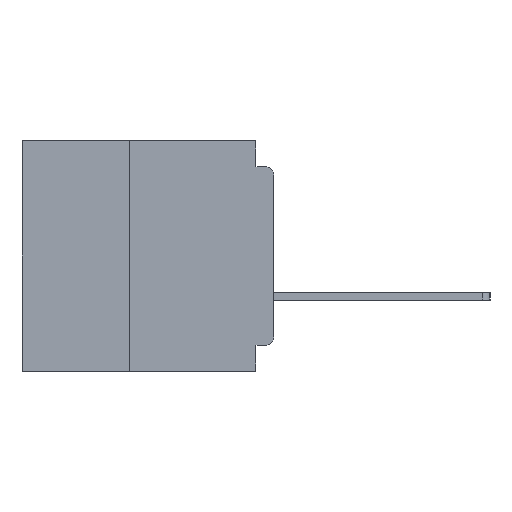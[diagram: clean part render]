
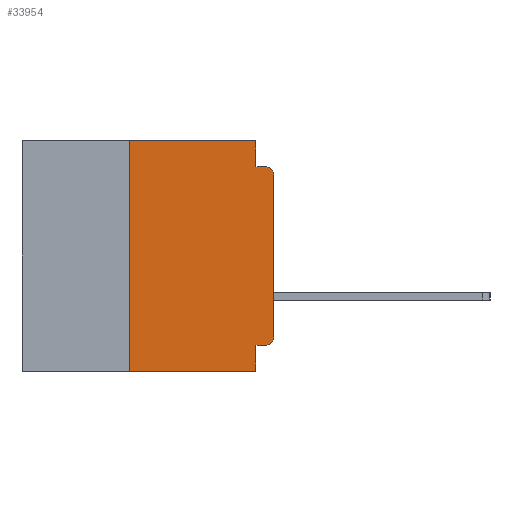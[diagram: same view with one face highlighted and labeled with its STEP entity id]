
A CAD part, left-side view. The second image highlights one B-rep face of the part: STEP entity #33954.
In plain terms, the highlighted planar face has unit normal (-1, 0, 0).
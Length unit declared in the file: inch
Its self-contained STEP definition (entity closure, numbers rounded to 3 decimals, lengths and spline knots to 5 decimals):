
#896 = CIRCLE ( 'NONE', #25414, 0.015 ) ;
#1188 = LINE ( 'NONE', #36605, #32529 ) ;
#1216 = EDGE_CURVE ( 'NONE', #43913, #44510, #28507, .T. ) ;
#1241 = ORIENTED_EDGE ( 'NONE', *, *, #37648, .T. ) ;
#2003 = ORIENTED_EDGE ( 'NONE', *, *, #7582, .T. ) ;
#2030 = DIRECTION ( 'NONE',  ( -1., 0., 0. ) ) ;
#2284 = FACE_OUTER_BOUND ( 'NONE', #9183, .T. ) ;
#2911 = DIRECTION ( 'NONE',  ( 0., 0., -1. ) ) ;
#6162 = CARTESIAN_POINT ( 'NONE',  ( 0., 0., -0.045 ) ) ;
#6522 = CARTESIAN_POINT ( 'NONE',  ( 0., 0.25, -0.4 ) ) ;
#6699 = LINE ( 'NONE', #11827, #48284 ) ;
#6799 = VERTEX_POINT ( 'NONE', #28355 ) ;
#6952 = VECTOR ( 'NONE', #48290, 39.37008 ) ;
#7582 = EDGE_CURVE ( 'NONE', #15148, #44510, #896, .T. ) ;
#9117 = DIRECTION ( 'NONE',  ( 0., 0., 1. ) ) ;
#9183 = EDGE_LOOP ( 'NONE', ( #1241, #2003, #47753, #50667, #33169, #31136, #35369, #17100, #23211, #42563 ) ) ;
#11827 = CARTESIAN_POINT ( 'NONE',  ( 0., 0., -0.355 ) ) ;
#12833 = DIRECTION ( 'NONE',  ( 0., 0., -1. ) ) ;
#12925 = VECTOR ( 'NONE', #45293, 39.37008 ) ;
#12945 = VERTEX_POINT ( 'NONE', #13798 ) ;
#13542 = DIRECTION ( 'NONE',  ( 0., 0., 1. ) ) ;
#13798 = CARTESIAN_POINT ( 'NONE',  ( 0., 0.25, 0. ) ) ;
#14037 = DIRECTION ( 'NONE',  ( 0., -1., 0. ) ) ;
#14270 = DIRECTION ( 'NONE',  ( 0., 0., -1. ) ) ;
#14556 = PLANE ( 'NONE',  #20321 ) ;
#15148 = VERTEX_POINT ( 'NONE', #35872 ) ;
#16348 = VERTEX_POINT ( 'NONE', #20618 ) ;
#16406 = EDGE_CURVE ( 'NONE', #37787, #12945, #1188, .T. ) ;
#17100 = ORIENTED_EDGE ( 'NONE', *, *, #24800, .F. ) ;
#17400 = LINE ( 'NONE', #20987, #6952 ) ;
#17873 = VERTEX_POINT ( 'NONE', #34628 ) ;
#18791 = VERTEX_POINT ( 'NONE', #40252 ) ;
#19396 = LINE ( 'NONE', #21833, #49317 ) ;
#19687 = CARTESIAN_POINT ( 'NONE',  ( 0., 0.015, -0.355 ) ) ;
#20256 = EDGE_CURVE ( 'NONE', #12945, #16348, #44165, .T. ) ;
#20321 = AXIS2_PLACEMENT_3D ( 'NONE', #49735, #26430, #2911 ) ;
#20618 = CARTESIAN_POINT ( 'NONE',  ( 0., 0.031, 0. ) ) ;
#20987 = CARTESIAN_POINT ( 'NONE',  ( 0., 0.437, -0.4 ) ) ;
#21560 = CARTESIAN_POINT ( 'NONE',  ( 0., 0.015, -0.34 ) ) ;
#21833 = CARTESIAN_POINT ( 'NONE',  ( 0., 0.031, 0. ) ) ;
#23211 = ORIENTED_EDGE ( 'NONE', *, *, #29988, .F. ) ;
#24709 = CARTESIAN_POINT ( 'NONE',  ( 0., 0.031, -0.4 ) ) ;
#24800 = EDGE_CURVE ( 'NONE', #18791, #6799, #26254, .T. ) ;
#25414 = AXIS2_PLACEMENT_3D ( 'NONE', #25529, #2030, #29526 ) ;
#25525 = DIRECTION ( 'NONE',  ( 0., 0., -1. ) ) ;
#25529 = CARTESIAN_POINT ( 'NONE',  ( 0., 0.015, -0.06 ) ) ;
#26254 = LINE ( 'NONE', #24709, #48163 ) ;
#26430 = DIRECTION ( 'NONE',  ( 1., 0., 0. ) ) ;
#27244 = EDGE_CURVE ( 'NONE', #42760, #17873, #44327, .T. ) ;
#28355 = CARTESIAN_POINT ( 'NONE',  ( 0., 0.031, -0.4 ) ) ;
#28507 = LINE ( 'NONE', #6162, #47971 ) ;
#29526 = DIRECTION ( 'NONE',  ( 0., 0., -1. ) ) ;
#29751 = AXIS2_PLACEMENT_3D ( 'NONE', #21560, #48847, #25525 ) ;
#29988 = EDGE_CURVE ( 'NONE', #42760, #18791, #6699, .T. ) ;
#31136 = ORIENTED_EDGE ( 'NONE', *, *, #16406, .F. ) ;
#32529 = VECTOR ( 'NONE', #9117, 39.37008 ) ;
#33169 = ORIENTED_EDGE ( 'NONE', *, *, #20256, .F. ) ;
#33179 = CARTESIAN_POINT ( 'NONE',  ( 0., 0., 0. ) ) ;
#33954 = ADVANCED_FACE ( 'NONE', ( #2284 ), #14556, .F. ) ;
#34628 = CARTESIAN_POINT ( 'NONE',  ( 0., 0., -0.34 ) ) ;
#35073 = EDGE_CURVE ( 'NONE', #16348, #43913, #19396, .T. ) ;
#35324 = CARTESIAN_POINT ( 'NONE',  ( 0., 0.015, -0.045 ) ) ;
#35369 = ORIENTED_EDGE ( 'NONE', *, *, #48543, .T. ) ;
#35555 = CARTESIAN_POINT ( 'NONE',  ( 0., 0.031, -0.045 ) ) ;
#35872 = CARTESIAN_POINT ( 'NONE',  ( 0., 0., -0.06 ) ) ;
#36605 = CARTESIAN_POINT ( 'NONE',  ( 0., 0.25, -0.4 ) ) ;
#37522 = CARTESIAN_POINT ( 'NONE',  ( 0., 0.437, 0. ) ) ;
#37648 = EDGE_CURVE ( 'NONE', #17873, #15148, #39985, .T. ) ;
#37787 = VERTEX_POINT ( 'NONE', #6522 ) ;
#38802 = VECTOR ( 'NONE', #13542, 39.37008 ) ;
#39256 = DIRECTION ( 'NONE',  ( 0., 1., 0. ) ) ;
#39985 = LINE ( 'NONE', #33179, #38802 ) ;
#40252 = CARTESIAN_POINT ( 'NONE',  ( 0., 0.031, -0.355 ) ) ;
#42563 = ORIENTED_EDGE ( 'NONE', *, *, #27244, .T. ) ;
#42760 = VERTEX_POINT ( 'NONE', #19687 ) ;
#43913 = VERTEX_POINT ( 'NONE', #35555 ) ;
#44165 = LINE ( 'NONE', #37522, #12925 ) ;
#44327 = CIRCLE ( 'NONE', #29751, 0.015 ) ;
#44510 = VERTEX_POINT ( 'NONE', #35324 ) ;
#45293 = DIRECTION ( 'NONE',  ( 0., -1., 0. ) ) ;
#47753 = ORIENTED_EDGE ( 'NONE', *, *, #1216, .F. ) ;
#47971 = VECTOR ( 'NONE', #14037, 39.37008 ) ;
#48163 = VECTOR ( 'NONE', #12833, 39.37008 ) ;
#48284 = VECTOR ( 'NONE', #39256, 39.37008 ) ;
#48290 = DIRECTION ( 'NONE',  ( 0., -1., 0. ) ) ;
#48543 = EDGE_CURVE ( 'NONE', #37787, #6799, #17400, .T. ) ;
#48847 = DIRECTION ( 'NONE',  ( -1., 0., 0. ) ) ;
#49317 = VECTOR ( 'NONE', #14270, 39.37008 ) ;
#49735 = CARTESIAN_POINT ( 'NONE',  ( 0., 0.437, 0. ) ) ;
#50667 = ORIENTED_EDGE ( 'NONE', *, *, #35073, .F. ) ;
